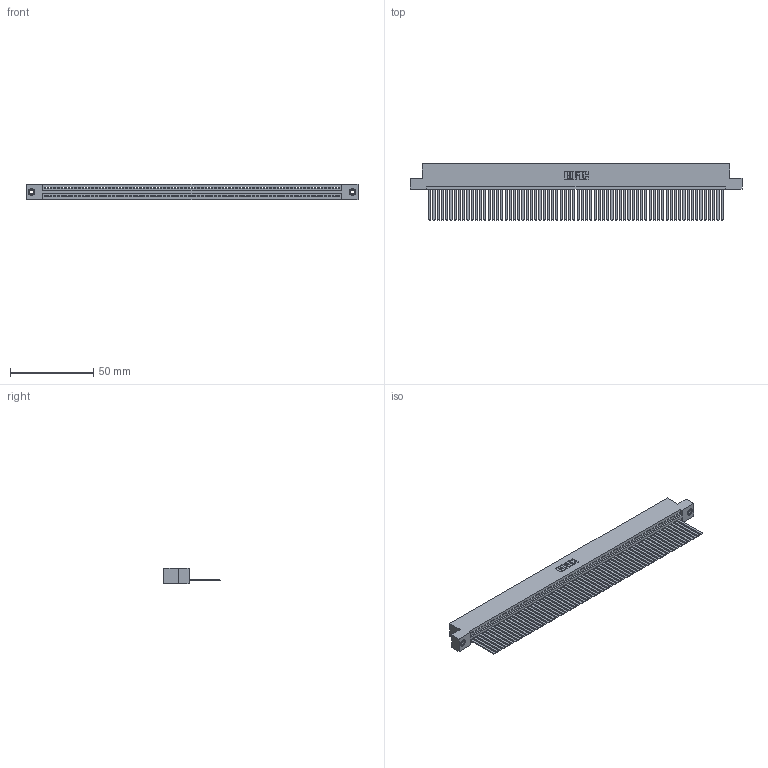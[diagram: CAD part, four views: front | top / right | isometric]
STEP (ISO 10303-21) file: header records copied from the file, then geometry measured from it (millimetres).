
FILE_DESCRIPTION (( 'STEP AP203' ), '1' );
FILE_NAME ('345-070-544-108.STEP', '2019-10-12T18:33:45', ( '' ), ( '' ), 'SwSTEP 2.0', 'SolidWorks 2016', '' );
FILE_SCHEMA (( 'CONFIG_CONTROL_DESIGN' ));
Length unit declared in the file: inch
Products named in the file (4): 345 Part_Flush Mounting Lugs - 0.156 Dia-TI; 345-292-001_345-293-144; 345-250-001_345-250-003-102; 345-070-544-108
Assembly tree (73 placements, depth 2):
  345-070-544-108
    345 Part_Flush Mounting Lugs - 0.156 Dia-TI
    345-292-001_345-293-144  x70
    345-250-001_345-250-003-102  x2
Bounding box: 199.01 x 33.96 x 9.4 mm (x, y, z)
Volume: 19935.6 mm3; surface area: 29326.1 mm2
Topology: 73 solids, 73 shells, 3826 faces, 11537 edges, 7590 vertices
Faces by surface type: plane 2632, cylinder 1178, cone 12, torus 4
Entity records: 49916 total; most frequent: CARTESIAN_POINT 8625, ORIENTED_EDGE 8622, DIRECTION 7517, EDGE_CURVE 4311, LINE 3883, VECTOR 3883, VERTEX_POINT 2868, AXIS2_PLACEMENT_3D 1817
